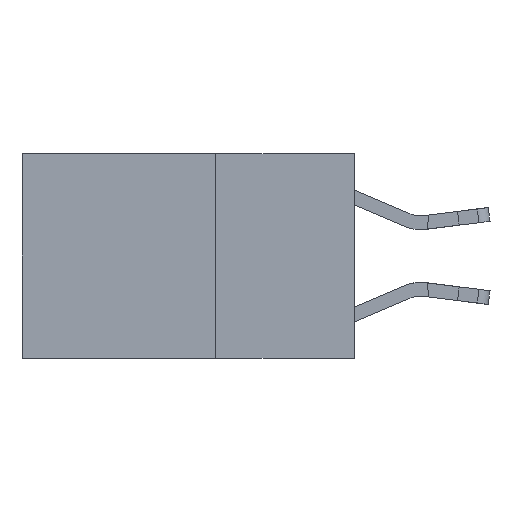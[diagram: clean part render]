
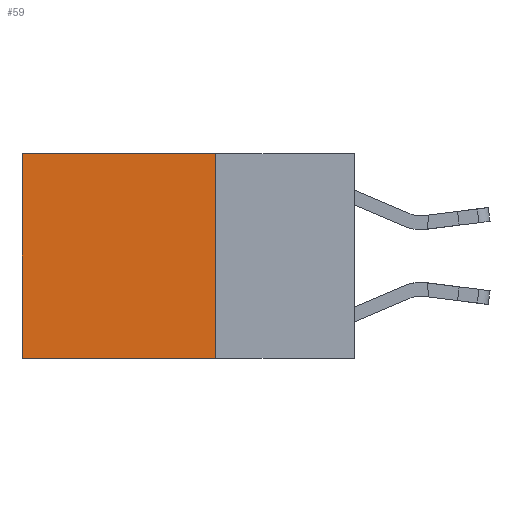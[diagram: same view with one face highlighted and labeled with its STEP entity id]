
A CAD part, left-side view. The second image highlights one B-rep face of the part: STEP entity #59.
In plain terms, the highlighted planar face has unit normal (-1, 0, 0).
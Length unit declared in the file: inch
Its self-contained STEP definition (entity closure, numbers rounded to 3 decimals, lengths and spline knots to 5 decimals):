
#59 = ADVANCED_FACE ( 'NONE', ( #8805 ), #8887, .F. ) ;
#211 = ORIENTED_EDGE ( 'NONE', *, *, #13187, .T. ) ;
#460 = CARTESIAN_POINT ( 'NONE',  ( 0.2625, 0.6, 0. ) ) ;
#602 = VECTOR ( 'NONE', #10933, 39.37008 ) ;
#605 = LINE ( 'NONE', #3946, #3085 ) ;
#1313 = VECTOR ( 'NONE', #9194, 39.37008 ) ;
#2065 = DIRECTION ( 'NONE',  ( 0., 1., 0. ) ) ;
#2168 = CARTESIAN_POINT ( 'NONE',  ( 0.2625, 0.25, 0. ) ) ;
#2819 = CARTESIAN_POINT ( 'NONE',  ( 0.2625, 0.25, -0.37 ) ) ;
#3085 = VECTOR ( 'NONE', #4026, 39.37008 ) ;
#3200 = CARTESIAN_POINT ( 'NONE',  ( 0.2625, 0.25, -0.37 ) ) ;
#3243 = EDGE_CURVE ( 'NONE', #4688, #5183, #4568, .T. ) ;
#3327 = LINE ( 'NONE', #10155, #602 ) ;
#3940 = CARTESIAN_POINT ( 'NONE',  ( 0.2625, 0.25, 0. ) ) ;
#3946 = CARTESIAN_POINT ( 'NONE',  ( 0.2625, 0.25, 0. ) ) ;
#4026 = DIRECTION ( 'NONE',  ( 0., 0., -1. ) ) ;
#4568 = LINE ( 'NONE', #3200, #9538 ) ;
#4688 = VERTEX_POINT ( 'NONE', #2819 ) ;
#4723 = VERTEX_POINT ( 'NONE', #460 ) ;
#4756 = EDGE_CURVE ( 'NONE', #10038, #4688, #605, .T. ) ;
#4989 = EDGE_LOOP ( 'NONE', ( #211, #10546, #13367, #11866 ) ) ;
#5183 = VERTEX_POINT ( 'NONE', #6435 ) ;
#5639 = AXIS2_PLACEMENT_3D ( 'NONE', #3940, #14401, #12274 ) ;
#6435 = CARTESIAN_POINT ( 'NONE',  ( 0.2625, 0.6, -0.37 ) ) ;
#6830 = LINE ( 'NONE', #10459, #1313 ) ;
#8805 = FACE_OUTER_BOUND ( 'NONE', #4989, .T. ) ;
#8887 = PLANE ( 'NONE',  #5639 ) ;
#9194 = DIRECTION ( 'NONE',  ( 0., 1., 0. ) ) ;
#9538 = VECTOR ( 'NONE', #2065, 39.37008 ) ;
#10038 = VERTEX_POINT ( 'NONE', #2168 ) ;
#10155 = CARTESIAN_POINT ( 'NONE',  ( 0.2625, 0.6, 0. ) ) ;
#10459 = CARTESIAN_POINT ( 'NONE',  ( 0.2625, 0.25, 0. ) ) ;
#10546 = ORIENTED_EDGE ( 'NONE', *, *, #3243, .F. ) ;
#10933 = DIRECTION ( 'NONE',  ( 0., 0., -1. ) ) ;
#11866 = ORIENTED_EDGE ( 'NONE', *, *, #12273, .T. ) ;
#12273 = EDGE_CURVE ( 'NONE', #10038, #4723, #6830, .T. ) ;
#12274 = DIRECTION ( 'NONE',  ( 0., 0., -1. ) ) ;
#13187 = EDGE_CURVE ( 'NONE', #4723, #5183, #3327, .T. ) ;
#13367 = ORIENTED_EDGE ( 'NONE', *, *, #4756, .F. ) ;
#14401 = DIRECTION ( 'NONE',  ( 1., 0., 0. ) ) ;
